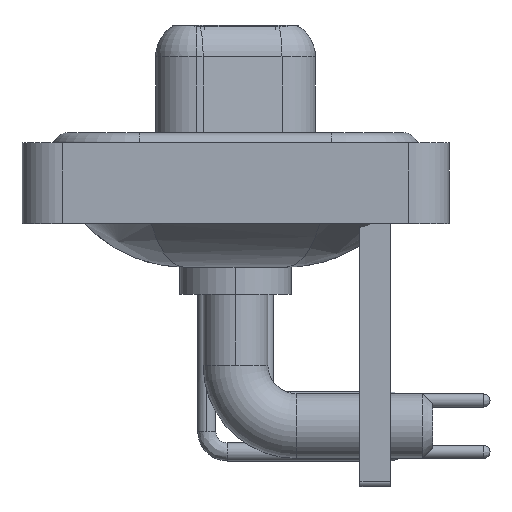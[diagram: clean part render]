
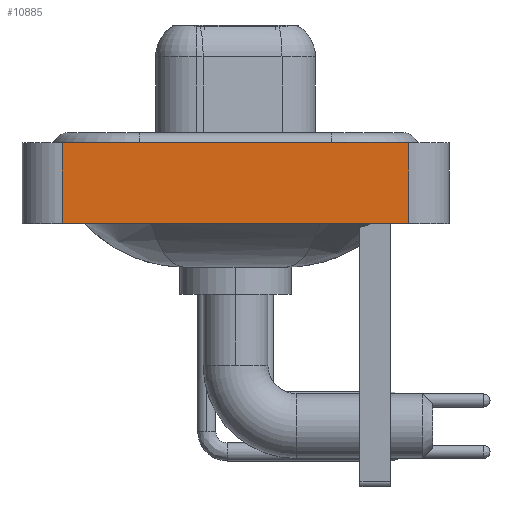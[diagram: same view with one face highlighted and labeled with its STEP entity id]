
A CAD part, left-side view. The second image highlights one B-rep face of the part: STEP entity #10885.
In plain terms, the highlighted planar face has unit normal (-1, 0, 0).
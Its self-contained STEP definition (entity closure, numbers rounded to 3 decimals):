
#458 = EDGE_LOOP ( 'NONE', ( #8988, #9885, #2338, #10001 ) ) ;
#1412 = VECTOR ( 'NONE', #7564, 1000. ) ;
#1852 = VERTEX_POINT ( 'NONE', #8647 ) ;
#2338 = ORIENTED_EDGE ( 'NONE', *, *, #11769, .F. ) ;
#2387 = CARTESIAN_POINT ( 'NONE',  ( -7.3, -8.55, -3.6 ) ) ;
#3110 = CARTESIAN_POINT ( 'NONE',  ( -7.3, 8.55, 0.4 ) ) ;
#3527 = EDGE_CURVE ( 'NONE', #19599, #16853, #12211, .T. ) ;
#4147 = DIRECTION ( 'NONE',  ( -1., 0., 0. ) ) ;
#4174 = CARTESIAN_POINT ( 'NONE',  ( -7.3, 8.55, -3.6 ) ) ;
#4594 = CARTESIAN_POINT ( 'NONE',  ( -7.3, -8.55, -3.6 ) ) ;
#5549 = DIRECTION ( 'NONE',  ( 0., 0., 1. ) ) ;
#6451 = LINE ( 'NONE', #13095, #19495 ) ;
#7564 = DIRECTION ( 'NONE',  ( 0., 0., 1. ) ) ;
#8647 = CARTESIAN_POINT ( 'NONE',  ( -7.3, 8.55, -3.6 ) ) ;
#8988 = ORIENTED_EDGE ( 'NONE', *, *, #3527, .T. ) ;
#9277 = FACE_OUTER_BOUND ( 'NONE', #458, .T. ) ;
#9885 = ORIENTED_EDGE ( 'NONE', *, *, #18801, .F. ) ;
#9936 = DIRECTION ( 'NONE',  ( 0., -1., 0. ) ) ;
#10001 = ORIENTED_EDGE ( 'NONE', *, *, #11575, .T. ) ;
#10244 = VECTOR ( 'NONE', #15284, 1000. ) ;
#10398 = LINE ( 'NONE', #17008, #10244 ) ;
#10800 = DIRECTION ( 'NONE',  ( 0., 0., 1. ) ) ;
#10885 = ADVANCED_FACE ( 'NONE', ( #9277 ), #15888, .T. ) ;
#11575 = EDGE_CURVE ( 'NONE', #1852, #19599, #10398, .T. ) ;
#11769 = EDGE_CURVE ( 'NONE', #1852, #17298, #14191, .T. ) ;
#12211 = LINE ( 'NONE', #13937, #21456 ) ;
#13095 = CARTESIAN_POINT ( 'NONE',  ( -7.3, -8.55, 0.4 ) ) ;
#13872 = CARTESIAN_POINT ( 'NONE',  ( -7.3, -8.55, 0.4 ) ) ;
#13937 = CARTESIAN_POINT ( 'NONE',  ( -7.3, -8.55, -3.6 ) ) ;
#14191 = LINE ( 'NONE', #4174, #1412 ) ;
#15284 = DIRECTION ( 'NONE',  ( 0., -1., 0. ) ) ;
#15888 = PLANE ( 'NONE',  #18146 ) ;
#16853 = VERTEX_POINT ( 'NONE', #13872 ) ;
#17008 = CARTESIAN_POINT ( 'NONE',  ( -7.3, -8.55, -3.6 ) ) ;
#17298 = VERTEX_POINT ( 'NONE', #3110 ) ;
#18146 = AXIS2_PLACEMENT_3D ( 'NONE', #4594, #4147, #10800 ) ;
#18801 = EDGE_CURVE ( 'NONE', #17298, #16853, #6451, .T. ) ;
#19495 = VECTOR ( 'NONE', #9936, 1000. ) ;
#19599 = VERTEX_POINT ( 'NONE', #2387 ) ;
#21456 = VECTOR ( 'NONE', #5549, 1000. ) ;
